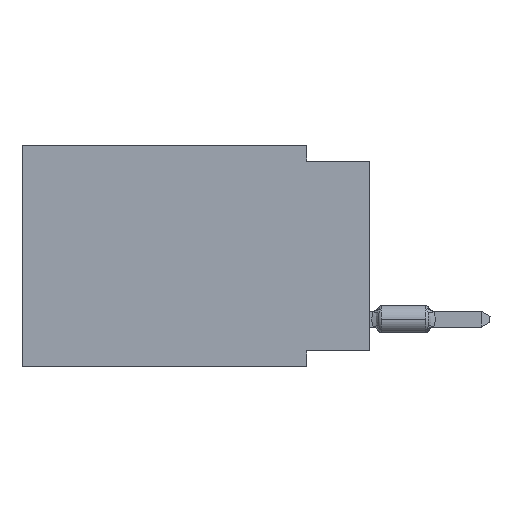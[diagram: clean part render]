
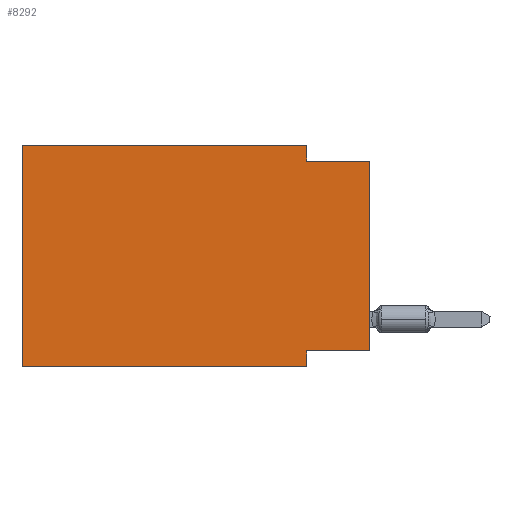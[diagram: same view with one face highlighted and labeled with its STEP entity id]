
A CAD part, left-side view. The second image highlights one B-rep face of the part: STEP entity #8292.
In plain terms, the highlighted planar face has unit normal (-1, 0, 0).
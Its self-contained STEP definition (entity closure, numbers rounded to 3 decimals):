
#1108 = VECTOR ( 'NONE', #14707, 1000. ) ;
#1205 = ORIENTED_EDGE ( 'NONE', *, *, #60992, .F. ) ;
#3245 = ORIENTED_EDGE ( 'NONE', *, *, #36438, .F. ) ;
#4958 = LINE ( 'NONE', #59396, #20303 ) ;
#5731 = VECTOR ( 'NONE', #39238, 1000. ) ;
#6981 = LINE ( 'NONE', #37911, #5731 ) ;
#7224 = DIRECTION ( 'NONE',  ( 0., 0., -1. ) ) ;
#8191 = VECTOR ( 'NONE', #14566, 1000. ) ;
#8292 = ADVANCED_FACE ( 'NONE', ( #55944 ), #12609, .F. ) ;
#9909 = CARTESIAN_POINT ( 'NONE',  ( 0., 13.97, -8.89 ) ) ;
#10197 = CARTESIAN_POINT ( 'NONE',  ( 0., 13.97, 0. ) ) ;
#12089 = VERTEX_POINT ( 'NONE', #60084 ) ;
#12609 = PLANE ( 'NONE',  #31707 ) ;
#13312 = CARTESIAN_POINT ( 'NONE',  ( 0., 13.97, 0. ) ) ;
#14566 = DIRECTION ( 'NONE',  ( 0., -1., 0. ) ) ;
#14707 = DIRECTION ( 'NONE',  ( 0., 0., -1. ) ) ;
#17742 = VERTEX_POINT ( 'NONE', #47376 ) ;
#19085 = VERTEX_POINT ( 'NONE', #10197 ) ;
#20291 = LINE ( 'NONE', #9909, #8191 ) ;
#20303 = VECTOR ( 'NONE', #32168, 1000. ) ;
#20922 = ORIENTED_EDGE ( 'NONE', *, *, #54749, .T. ) ;
#23886 = DIRECTION ( 'NONE',  ( 0., 0., 1. ) ) ;
#23915 = VECTOR ( 'NONE', #30191, 1000. ) ;
#24299 = EDGE_CURVE ( 'NONE', #26201, #40863, #67746, .T. ) ;
#24506 = VECTOR ( 'NONE', #26177, 1000. ) ;
#26177 = DIRECTION ( 'NONE',  ( 0., 0., 1. ) ) ;
#26201 = VERTEX_POINT ( 'NONE', #43215 ) ;
#27949 = ORIENTED_EDGE ( 'NONE', *, *, #48830, .T. ) ;
#28896 = VERTEX_POINT ( 'NONE', #63934 ) ;
#30191 = DIRECTION ( 'NONE',  ( 0., -1., 0. ) ) ;
#30203 = ORIENTED_EDGE ( 'NONE', *, *, #53245, .F. ) ;
#30661 = LINE ( 'NONE', #51462, #38050 ) ;
#31707 = AXIS2_PLACEMENT_3D ( 'NONE', #13312, #35150, #7224 ) ;
#31898 = LINE ( 'NONE', #54098, #24506 ) ;
#32168 = DIRECTION ( 'NONE',  ( 0., 0., -1. ) ) ;
#35150 = DIRECTION ( 'NONE',  ( 1., 0., 0. ) ) ;
#35562 = LINE ( 'NONE', #36987, #23915 ) ;
#36438 = EDGE_CURVE ( 'NONE', #12089, #26201, #50513, .T. ) ;
#36987 = CARTESIAN_POINT ( 'NONE',  ( 0., 0., -0.635 ) ) ;
#37911 = CARTESIAN_POINT ( 'NONE',  ( 0., 13.97, 0. ) ) ;
#38050 = VECTOR ( 'NONE', #23886, 1000. ) ;
#39238 = DIRECTION ( 'NONE',  ( 0., -1., 0. ) ) ;
#40504 = DIRECTION ( 'NONE',  ( 0., 1., 0. ) ) ;
#40863 = VERTEX_POINT ( 'NONE', #51711 ) ;
#43153 = VERTEX_POINT ( 'NONE', #66589 ) ;
#43215 = CARTESIAN_POINT ( 'NONE',  ( 0., 2.54, -8.255 ) ) ;
#43767 = ORIENTED_EDGE ( 'NONE', *, *, #24299, .F. ) ;
#44414 = EDGE_LOOP ( 'NONE', ( #27949, #47937, #1205, #30203, #70592, #20922, #43767, #3245 ) ) ;
#46456 = CARTESIAN_POINT ( 'NONE',  ( 0., 13.97, -8.89 ) ) ;
#47376 = CARTESIAN_POINT ( 'NONE',  ( 0., 2.54, -0.635 ) ) ;
#47937 = ORIENTED_EDGE ( 'NONE', *, *, #70382, .F. ) ;
#48830 = EDGE_CURVE ( 'NONE', #12089, #28896, #30661, .T. ) ;
#50513 = LINE ( 'NONE', #61990, #51106 ) ;
#51106 = VECTOR ( 'NONE', #40504, 1000. ) ;
#51462 = CARTESIAN_POINT ( 'NONE',  ( 0., 0., 0. ) ) ;
#51711 = CARTESIAN_POINT ( 'NONE',  ( 0., 2.54, -8.89 ) ) ;
#53245 = EDGE_CURVE ( 'NONE', #19085, #43153, #6981, .T. ) ;
#54098 = CARTESIAN_POINT ( 'NONE',  ( 0., 13.97, 0. ) ) ;
#54749 = EDGE_CURVE ( 'NONE', #61263, #40863, #20291, .T. ) ;
#55944 = FACE_OUTER_BOUND ( 'NONE', #44414, .T. ) ;
#56979 = CARTESIAN_POINT ( 'NONE',  ( 0., 2.54, -8.89 ) ) ;
#59396 = CARTESIAN_POINT ( 'NONE',  ( 0., 2.54, 0. ) ) ;
#60084 = CARTESIAN_POINT ( 'NONE',  ( 0., 0., -8.255 ) ) ;
#60992 = EDGE_CURVE ( 'NONE', #43153, #17742, #4958, .T. ) ;
#61263 = VERTEX_POINT ( 'NONE', #46456 ) ;
#61990 = CARTESIAN_POINT ( 'NONE',  ( 0., 0., -8.255 ) ) ;
#63934 = CARTESIAN_POINT ( 'NONE',  ( 0., 0., -0.635 ) ) ;
#65616 = EDGE_CURVE ( 'NONE', #61263, #19085, #31898, .T. ) ;
#66589 = CARTESIAN_POINT ( 'NONE',  ( 0., 2.54, 0. ) ) ;
#67746 = LINE ( 'NONE', #56979, #1108 ) ;
#70382 = EDGE_CURVE ( 'NONE', #17742, #28896, #35562, .T. ) ;
#70592 = ORIENTED_EDGE ( 'NONE', *, *, #65616, .F. ) ;
